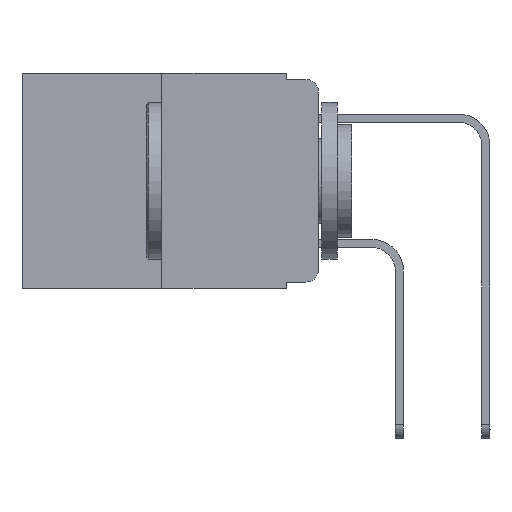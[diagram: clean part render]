
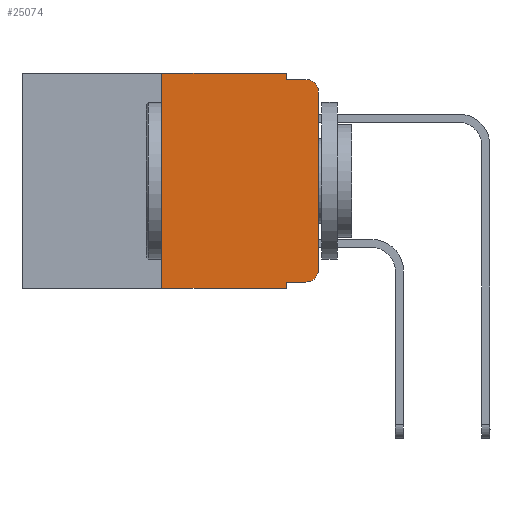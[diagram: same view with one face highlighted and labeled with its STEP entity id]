
A CAD part, left-side view. The second image highlights one B-rep face of the part: STEP entity #25074.
In plain terms, the highlighted planar face has unit normal (-1, 0, 0).
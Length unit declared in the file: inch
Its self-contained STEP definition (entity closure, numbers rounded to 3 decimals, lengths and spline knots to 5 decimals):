
#21 = EDGE_CURVE ( 'NONE', #15060, #10422, #11957, .T. ) ;
#28 = VECTOR ( 'NONE', #7391, 39.37008 ) ;
#74 = DIRECTION ( 'NONE',  ( -1., 0., 0. ) ) ;
#282 = CARTESIAN_POINT ( 'NONE',  ( 0., 0., -0.313 ) ) ;
#408 = CARTESIAN_POINT ( 'NONE',  ( 0., 0.051, 0. ) ) ;
#466 = LINE ( 'NONE', #8686, #21633 ) ;
#471 = VECTOR ( 'NONE', #8491, 39.37008 ) ;
#1129 = EDGE_CURVE ( 'NONE', #14794, #12770, #10566, .T. ) ;
#1169 = CARTESIAN_POINT ( 'NONE',  ( 0., 0.473, -0.343 ) ) ;
#1350 = CARTESIAN_POINT ( 'NONE',  ( 0., 0.473, 0. ) ) ;
#1533 = DIRECTION ( 'NONE',  ( 0., 0., -1. ) ) ;
#2371 = VERTEX_POINT ( 'NONE', #17833 ) ;
#2912 = LINE ( 'NONE', #16906, #10405 ) ;
#3756 = CARTESIAN_POINT ( 'NONE',  ( 0., 0.02, -0.01 ) ) ;
#3821 = EDGE_CURVE ( 'NONE', #19318, #2371, #20598, .T. ) ;
#4183 = DIRECTION ( 'NONE',  ( -1., 0., 0. ) ) ;
#6510 = ORIENTED_EDGE ( 'NONE', *, *, #3821, .F. ) ;
#6567 = ORIENTED_EDGE ( 'NONE', *, *, #23092, .F. ) ;
#6610 = CARTESIAN_POINT ( 'NONE',  ( 0., 0.25, 0. ) ) ;
#6683 = CARTESIAN_POINT ( 'NONE',  ( 0., 0., 0. ) ) ;
#7391 = DIRECTION ( 'NONE',  ( 0., 0., -1. ) ) ;
#7640 = ORIENTED_EDGE ( 'NONE', *, *, #21, .T. ) ;
#7771 = DIRECTION ( 'NONE',  ( 1., 0., 0. ) ) ;
#7797 = ORIENTED_EDGE ( 'NONE', *, *, #11297, .T. ) ;
#8378 = AXIS2_PLACEMENT_3D ( 'NONE', #11484, #7771, #21488 ) ;
#8491 = DIRECTION ( 'NONE',  ( 0., 0., -1. ) ) ;
#8686 = CARTESIAN_POINT ( 'NONE',  ( 0., 0.25, 0. ) ) ;
#8876 = DIRECTION ( 'NONE',  ( 0., -1., 0. ) ) ;
#9325 = EDGE_CURVE ( 'NONE', #14794, #22775, #25081, .T. ) ;
#9390 = VERTEX_POINT ( 'NONE', #17149 ) ;
#9461 = ORIENTED_EDGE ( 'NONE', *, *, #9325, .F. ) ;
#10017 = ORIENTED_EDGE ( 'NONE', *, *, #11395, .T. ) ;
#10018 = VECTOR ( 'NONE', #19571, 39.37008 ) ;
#10038 = CARTESIAN_POINT ( 'NONE',  ( 0., 0.02, -0.333 ) ) ;
#10271 = LINE ( 'NONE', #6683, #25025 ) ;
#10405 = VECTOR ( 'NONE', #20726, 39.37008 ) ;
#10422 = VERTEX_POINT ( 'NONE', #3756 ) ;
#10566 = LINE ( 'NONE', #18451, #21475 ) ;
#10682 = VECTOR ( 'NONE', #8876, 39.37008 ) ;
#10975 = CARTESIAN_POINT ( 'NONE',  ( 0., 0.051, 0. ) ) ;
#11297 = EDGE_CURVE ( 'NONE', #12770, #23051, #23712, .T. ) ;
#11357 = EDGE_CURVE ( 'NONE', #9390, #24980, #466, .T. ) ;
#11395 = EDGE_CURVE ( 'NONE', #23051, #15060, #10271, .T. ) ;
#11420 = LINE ( 'NONE', #1350, #10018 ) ;
#11484 = CARTESIAN_POINT ( 'NONE',  ( 0., 0.473, 0. ) ) ;
#11957 = CIRCLE ( 'NONE', #25438, 0.02 ) ;
#11985 = CARTESIAN_POINT ( 'NONE',  ( 0., 0.02, -0.03 ) ) ;
#12356 = AXIS2_PLACEMENT_3D ( 'NONE', #24240, #4183, #19261 ) ;
#12374 = EDGE_CURVE ( 'NONE', #9390, #22775, #12690, .T. ) ;
#12690 = LINE ( 'NONE', #1169, #10682 ) ;
#12770 = VERTEX_POINT ( 'NONE', #10038 ) ;
#13758 = CARTESIAN_POINT ( 'NONE',  ( 0., 0.051, -0.343 ) ) ;
#14320 = CARTESIAN_POINT ( 'NONE',  ( 0., 0., -0.03 ) ) ;
#14794 = VERTEX_POINT ( 'NONE', #17359 ) ;
#14854 = DIRECTION ( 'NONE',  ( 0., 0., 1. ) ) ;
#15005 = ORIENTED_EDGE ( 'NONE', *, *, #24231, .F. ) ;
#15060 = VERTEX_POINT ( 'NONE', #14320 ) ;
#16198 = EDGE_LOOP ( 'NONE', ( #10017, #7640, #6567, #6510, #15005, #20876, #24019, #9461, #23420, #7797 ) ) ;
#16600 = DIRECTION ( 'NONE',  ( 0., -1., 0. ) ) ;
#16906 = CARTESIAN_POINT ( 'NONE',  ( 0., 0.051, -0.01 ) ) ;
#17149 = CARTESIAN_POINT ( 'NONE',  ( 0., 0.25, -0.343 ) ) ;
#17359 = CARTESIAN_POINT ( 'NONE',  ( 0., 0.051, -0.333 ) ) ;
#17833 = CARTESIAN_POINT ( 'NONE',  ( 0., 0.051, -0.01 ) ) ;
#18451 = CARTESIAN_POINT ( 'NONE',  ( 0., 0.051, -0.333 ) ) ;
#19253 = PLANE ( 'NONE',  #8378 ) ;
#19261 = DIRECTION ( 'NONE',  ( 0., 0., -1. ) ) ;
#19318 = VERTEX_POINT ( 'NONE', #25739 ) ;
#19571 = DIRECTION ( 'NONE',  ( 0., -1., 0. ) ) ;
#20408 = DIRECTION ( 'NONE',  ( 0., 0., 1. ) ) ;
#20598 = LINE ( 'NONE', #408, #471 ) ;
#20726 = DIRECTION ( 'NONE',  ( 0., -1., 0. ) ) ;
#20876 = ORIENTED_EDGE ( 'NONE', *, *, #11357, .F. ) ;
#21475 = VECTOR ( 'NONE', #16600, 39.37008 ) ;
#21488 = DIRECTION ( 'NONE',  ( 0., 0., -1. ) ) ;
#21633 = VECTOR ( 'NONE', #20408, 39.37008 ) ;
#21875 = FACE_OUTER_BOUND ( 'NONE', #16198, .T. ) ;
#22775 = VERTEX_POINT ( 'NONE', #13758 ) ;
#23051 = VERTEX_POINT ( 'NONE', #282 ) ;
#23092 = EDGE_CURVE ( 'NONE', #2371, #10422, #2912, .T. ) ;
#23420 = ORIENTED_EDGE ( 'NONE', *, *, #1129, .T. ) ;
#23712 = CIRCLE ( 'NONE', #12356, 0.02 ) ;
#24019 = ORIENTED_EDGE ( 'NONE', *, *, #12374, .T. ) ;
#24231 = EDGE_CURVE ( 'NONE', #24980, #19318, #11420, .T. ) ;
#24240 = CARTESIAN_POINT ( 'NONE',  ( 0., 0.02, -0.313 ) ) ;
#24980 = VERTEX_POINT ( 'NONE', #6610 ) ;
#25025 = VECTOR ( 'NONE', #14854, 39.37008 ) ;
#25074 = ADVANCED_FACE ( 'NONE', ( #21875 ), #19253, .F. ) ;
#25081 = LINE ( 'NONE', #10975, #28 ) ;
#25438 = AXIS2_PLACEMENT_3D ( 'NONE', #11985, #74, #1533 ) ;
#25739 = CARTESIAN_POINT ( 'NONE',  ( 0., 0.051, 0. ) ) ;
